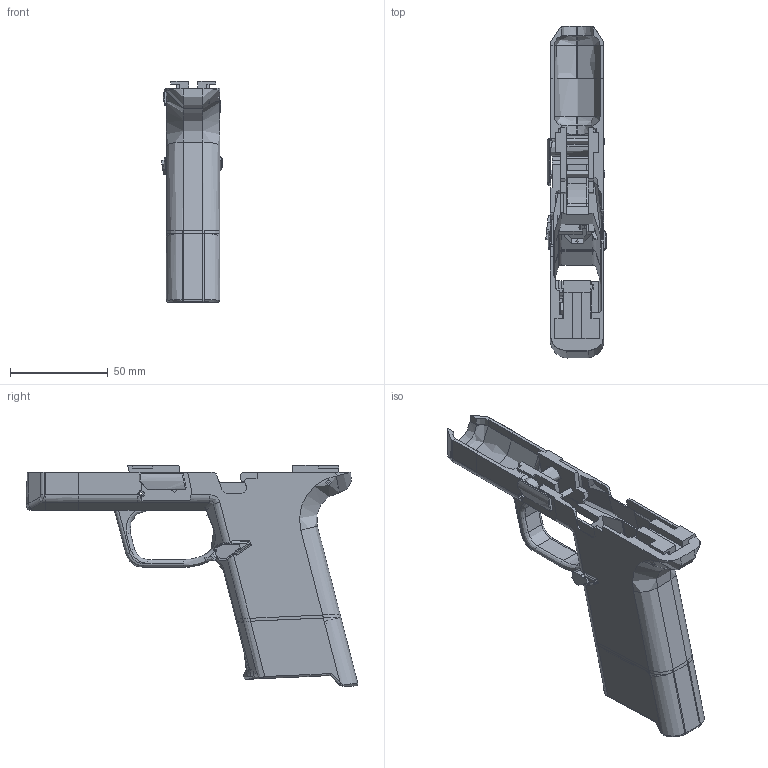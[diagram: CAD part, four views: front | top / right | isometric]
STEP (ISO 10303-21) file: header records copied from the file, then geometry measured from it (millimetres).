
FILE_DESCRIPTION(/* description */ (''),/* implementation_level */ '2;1');
FILE_NAME(/* name */ 'M&P 9 Assembly.step',/* time_stamp */ '2021-12-25T22:48:18-05:00',/* author */ (''),/* organization */ (''),/* preprocessor_version */ 'ST-DEVELOPER v18.1',/* originating_system */ 'Autodesk Translation Framework v10.10.0.1391',/* authorisation */ '');
FILE_SCHEMA (('AUTOMOTIVE_DESIGN { 1 0 10303 214 3 1 1 }'));
Length unit declared in the file: millimetre
Products named in the file (13): M&P 9 Reference; Rear Fire Control Group Pin; Front Locking Block Group Pin; Trigger Pin; Locking Block; Disassembly Lug; Rear Fire Control Group; Frame; Trigger Guard and Magwell; Fitment Section; Nose; Full-Size Magwell Body; Magazine Release Button
Assembly tree (12 placements, depth 4):
  M&P 9 Reference
    Rear Fire Control Group Pin
    Front Locking Block Group Pin
    Trigger Pin
    Locking Block
    Disassembly Lug
    Rear Fire Control Group
    Frame
      Trigger Guard and Magwell
      Fitment Section
        Nose
      Full-Size Magwell Body
    Magazine Release Button
Bounding box: 30.95 x 169.75 x 113.13 mm (x, y, z)
Volume: 102943 mm3; surface area: 57786.9 mm2
Topology: 12 solids, 12 shells, 695 faces, 1881 edges, 1195 vertices
Faces by surface type: plane 349, cylinder 205, bspline 113, torus 21, sphere 4, cone 3
Full cylindrical faces by diameter (mm): 1.35 x2, 1.5 x3, 3 x1, 3.15 x2, 3.18 x3, 3.2 x2, 3.361 x2, 3.5 x1, 3.55 x4, 4.7 x1, 5.1 x1, 6.3 x1, 7.7 x1, 8.8 x1, 9 x2
Entity records: 25989 total; most frequent: CARTESIAN_POINT 8438, ORIENTED_EDGE 3740, DIRECTION 3407, EDGE_CURVE 1870, VERTEX_POINT 1195, AXIS2_PLACEMENT_3D 1146, LINE 1115, VECTOR 1115
